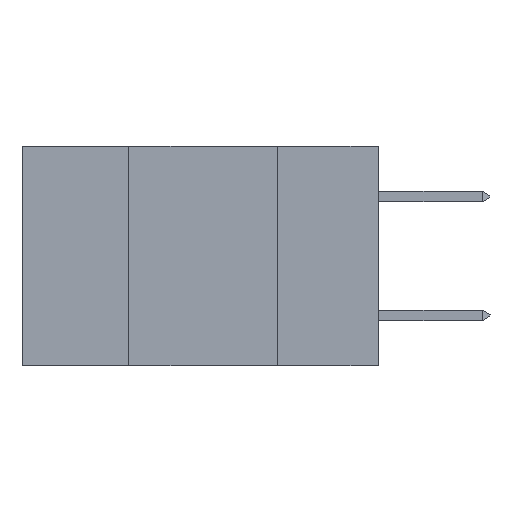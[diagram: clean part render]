
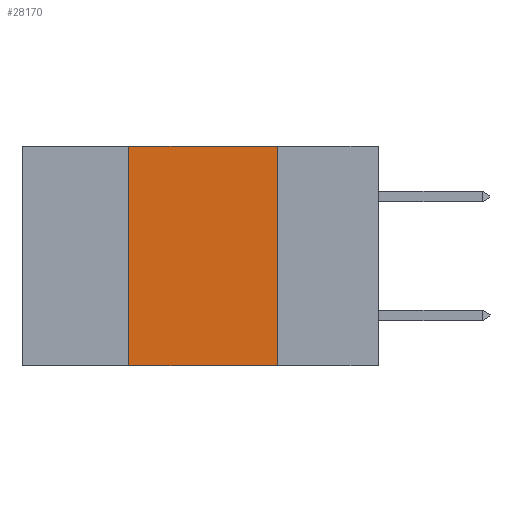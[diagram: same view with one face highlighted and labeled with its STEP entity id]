
A CAD part, left-side view. The second image highlights one B-rep face of the part: STEP entity #28170.
In plain terms, the highlighted planar face has unit normal (-1, 0, 0).
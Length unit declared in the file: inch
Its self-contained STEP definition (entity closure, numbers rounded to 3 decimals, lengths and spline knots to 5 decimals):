
#83 = LINE ( 'NONE', #24608, #10833 ) ;
#401 = ORIENTED_EDGE ( 'NONE', *, *, #8761, .F. ) ;
#907 = CARTESIAN_POINT ( 'NONE',  ( 0., 0.6, 0. ) ) ;
#1646 = EDGE_CURVE ( 'NONE', #10059, #7648, #12023, .T. ) ;
#4526 = VECTOR ( 'NONE', #19598, 39.37008 ) ;
#5244 = AXIS2_PLACEMENT_3D ( 'NONE', #6697, #27102, #13445 ) ;
#5596 = VECTOR ( 'NONE', #9269, 39.37008 ) ;
#5892 = EDGE_CURVE ( 'NONE', #6006, #26488, #14532, .T. ) ;
#6006 = VERTEX_POINT ( 'NONE', #29383 ) ;
#6697 = CARTESIAN_POINT ( 'NONE',  ( 0., 0.6, 0. ) ) ;
#7648 = VERTEX_POINT ( 'NONE', #23730 ) ;
#8761 = EDGE_CURVE ( 'NONE', #6006, #10059, #83, .T. ) ;
#9269 = DIRECTION ( 'NONE',  ( 0., -1., 0. ) ) ;
#10059 = VERTEX_POINT ( 'NONE', #13474 ) ;
#10833 = VECTOR ( 'NONE', #24989, 39.37008 ) ;
#12023 = LINE ( 'NONE', #907, #5596 ) ;
#13445 = DIRECTION ( 'NONE',  ( 0., 0., -1. ) ) ;
#13474 = CARTESIAN_POINT ( 'NONE',  ( 0., 0.42, 0. ) ) ;
#14532 = LINE ( 'NONE', #17182, #4526 ) ;
#16422 = ORIENTED_EDGE ( 'NONE', *, *, #1646, .F. ) ;
#17182 = CARTESIAN_POINT ( 'NONE',  ( 0., 0.6, -0.37 ) ) ;
#17249 = EDGE_LOOP ( 'NONE', ( #22227, #16422, #401, #21362 ) ) ;
#18011 = PLANE ( 'NONE',  #5244 ) ;
#18522 = EDGE_CURVE ( 'NONE', #7648, #26488, #29382, .T. ) ;
#19598 = DIRECTION ( 'NONE',  ( 0., -1., 0. ) ) ;
#21032 = FACE_OUTER_BOUND ( 'NONE', #17249, .T. ) ;
#21362 = ORIENTED_EDGE ( 'NONE', *, *, #5892, .T. ) ;
#21422 = DIRECTION ( 'NONE',  ( 0., 0., -1. ) ) ;
#22227 = ORIENTED_EDGE ( 'NONE', *, *, #18522, .F. ) ;
#23485 = CARTESIAN_POINT ( 'NONE',  ( 0., 0.17, -0.37 ) ) ;
#23730 = CARTESIAN_POINT ( 'NONE',  ( 0., 0.17, 0. ) ) ;
#24093 = VECTOR ( 'NONE', #21422, 39.37008 ) ;
#24608 = CARTESIAN_POINT ( 'NONE',  ( 0., 0.42, 0. ) ) ;
#24989 = DIRECTION ( 'NONE',  ( 0., 0., 1. ) ) ;
#26022 = CARTESIAN_POINT ( 'NONE',  ( 0., 0.17, 0. ) ) ;
#26488 = VERTEX_POINT ( 'NONE', #23485 ) ;
#27102 = DIRECTION ( 'NONE',  ( 1., 0., 0. ) ) ;
#28170 = ADVANCED_FACE ( 'NONE', ( #21032 ), #18011, .F. ) ;
#29382 = LINE ( 'NONE', #26022, #24093 ) ;
#29383 = CARTESIAN_POINT ( 'NONE',  ( 0., 0.42, -0.37 ) ) ;
